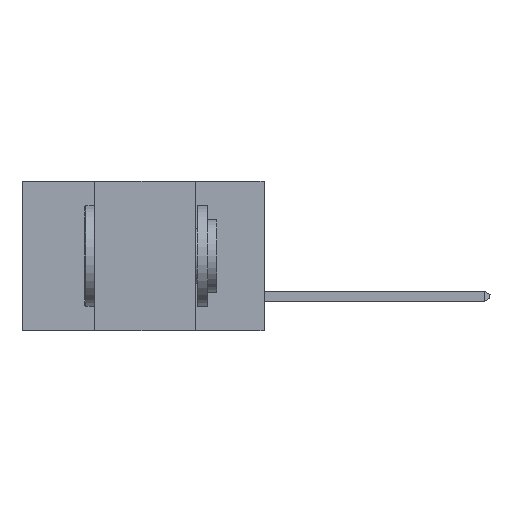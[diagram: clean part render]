
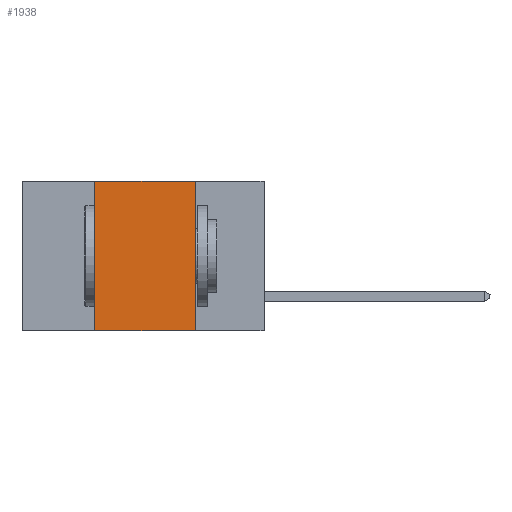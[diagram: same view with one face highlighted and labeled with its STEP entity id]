
A CAD part, left-side view. The second image highlights one B-rep face of the part: STEP entity #1938.
In plain terms, the highlighted planar face has unit normal (-1, 0, 0).
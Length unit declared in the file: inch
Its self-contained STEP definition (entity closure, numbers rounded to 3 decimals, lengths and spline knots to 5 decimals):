
#73 = EDGE_CURVE ( 'NONE', #10135, #3957, #19773, .T. ) ;
#269 = VECTOR ( 'NONE', #7350, 39.37008 ) ;
#337 = CARTESIAN_POINT ( 'NONE',  ( 0., 0.6, -0.37 ) ) ;
#887 = LINE ( 'NONE', #10071, #269 ) ;
#1938 = ADVANCED_FACE ( 'NONE', ( #24047 ), #10480, .F. ) ;
#2233 = VERTEX_POINT ( 'NONE', #7108 ) ;
#2476 = DIRECTION ( 'NONE',  ( 1., 0., 0. ) ) ;
#2544 = EDGE_CURVE ( 'NONE', #15969, #3957, #12482, .T. ) ;
#2648 = DIRECTION ( 'NONE',  ( 0., 0., -1. ) ) ;
#3238 = ORIENTED_EDGE ( 'NONE', *, *, #11139, .F. ) ;
#3812 = DIRECTION ( 'NONE',  ( 0., 0., -1. ) ) ;
#3957 = VERTEX_POINT ( 'NONE', #9266 ) ;
#5390 = VECTOR ( 'NONE', #3812, 39.37008 ) ;
#5561 = DIRECTION ( 'NONE',  ( 0., -1., 0. ) ) ;
#5630 = CARTESIAN_POINT ( 'NONE',  ( 0., 0.6, 0. ) ) ;
#6473 = DIRECTION ( 'NONE',  ( 0., -1., 0. ) ) ;
#6622 = CARTESIAN_POINT ( 'NONE',  ( 0., 0.6, 0. ) ) ;
#7108 = CARTESIAN_POINT ( 'NONE',  ( 0., 0.42, 0. ) ) ;
#7350 = DIRECTION ( 'NONE',  ( 0., 0., 1. ) ) ;
#7400 = VECTOR ( 'NONE', #5561, 39.37008 ) ;
#7687 = CARTESIAN_POINT ( 'NONE',  ( 0., 0.17, 0. ) ) ;
#9214 = ORIENTED_EDGE ( 'NONE', *, *, #16207, .F. ) ;
#9266 = CARTESIAN_POINT ( 'NONE',  ( 0., 0.17, -0.37 ) ) ;
#9289 = LINE ( 'NONE', #5630, #7400 ) ;
#10071 = CARTESIAN_POINT ( 'NONE',  ( 0., 0.42, 0. ) ) ;
#10135 = VERTEX_POINT ( 'NONE', #14380 ) ;
#10480 = PLANE ( 'NONE',  #19379 ) ;
#11139 = EDGE_CURVE ( 'NONE', #2233, #10135, #9289, .T. ) ;
#12482 = LINE ( 'NONE', #337, #17125 ) ;
#14380 = CARTESIAN_POINT ( 'NONE',  ( 0., 0.17, 0. ) ) ;
#15202 = ORIENTED_EDGE ( 'NONE', *, *, #2544, .T. ) ;
#15969 = VERTEX_POINT ( 'NONE', #23436 ) ;
#16207 = EDGE_CURVE ( 'NONE', #15969, #2233, #887, .T. ) ;
#16990 = EDGE_LOOP ( 'NONE', ( #17133, #3238, #9214, #15202 ) ) ;
#17125 = VECTOR ( 'NONE', #6473, 39.37008 ) ;
#17133 = ORIENTED_EDGE ( 'NONE', *, *, #73, .F. ) ;
#19379 = AXIS2_PLACEMENT_3D ( 'NONE', #6622, #2476, #2648 ) ;
#19773 = LINE ( 'NONE', #7687, #5390 ) ;
#23436 = CARTESIAN_POINT ( 'NONE',  ( 0., 0.42, -0.37 ) ) ;
#24047 = FACE_OUTER_BOUND ( 'NONE', #16990, .T. ) ;
